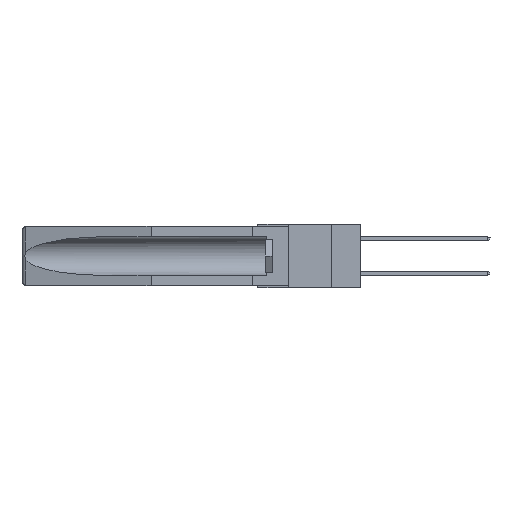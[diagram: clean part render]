
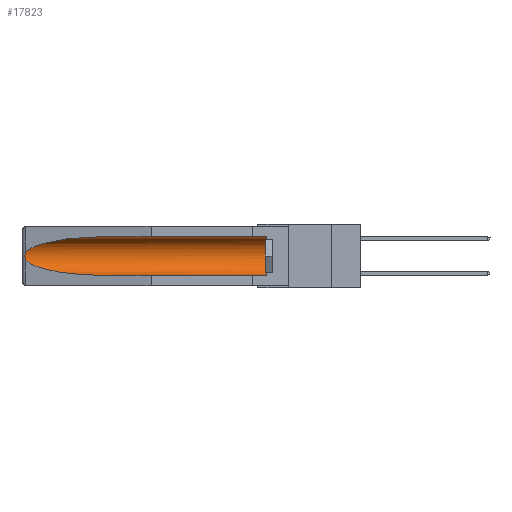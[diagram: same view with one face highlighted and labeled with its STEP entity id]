
A CAD part, left-side view. The second image highlights one B-rep face of the part: STEP entity #17823.
In plain terms, the highlighted cylindrical face has radius 2.857 mm (diameter 5.715 mm), a partial arc.
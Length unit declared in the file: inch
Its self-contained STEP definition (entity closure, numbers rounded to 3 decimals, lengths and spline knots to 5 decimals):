
#705 = DIRECTION ( 'NONE',  ( 0., -1., 0. ) ) ;
#1316 = CARTESIAN_POINT ( 'NONE',  ( 0.26537, 1.52718, -0.14972 ) ) ;
#1334 = VERTEX_POINT ( 'NONE', #18808 ) ;
#1489 = CARTESIAN_POINT ( 'NONE',  ( 0.2673, 1.5327, -0.16383 ) ) ;
#1999 = CARTESIAN_POINT ( 'NONE',  ( 0.155, 1.07973, -0.059 ) ) ;
#2081 = ORIENTED_EDGE ( 'NONE', *, *, #20982, .T. ) ;
#2221 = CARTESIAN_POINT ( 'NONE',  ( 0.155, -0.30754, -0.059 ) ) ;
#3164 = ORIENTED_EDGE ( 'NONE', *, *, #6836, .T. ) ;
#3399 = CARTESIAN_POINT ( 'NONE',  ( 0.2675, 1.53308, -0.16763 ) ) ;
#3469 = CARTESIAN_POINT ( 'NONE',  ( 0.2675, 1.53308, -0.17534 ) ) ;
#3472 = CARTESIAN_POINT ( 'NONE',  ( 0.155, 1.07973, -0.284 ) ) ;
#4184 = CARTESIAN_POINT ( 'NONE',  ( 0.155, -0.30754, -0.284 ) ) ;
#4378 = VERTEX_POINT ( 'NONE', #1999 ) ;
#4438 = CARTESIAN_POINT ( 'NONE',  ( 0.155, -0.30754, -0.1715 ) ) ;
#5436 = CARTESIAN_POINT ( 'NONE',  ( 0.2673, 1.53269, -0.17917 ) ) ;
#5707 =( BOUNDED_CURVE ( )  B_SPLINE_CURVE ( 3, ( #8137, #16280, #16543, #6509 ),
 .UNSPECIFIED., .F., .F. ) 
 B_SPLINE_CURVE_WITH_KNOTS ( ( 4, 4 ),
 ( 0.1948, 1.5708 ),
 .UNSPECIFIED. ) 
 CURVE ( )  GEOMETRIC_REPRESENTATION_ITEM ( )  RATIONAL_B_SPLINE_CURVE ( ( 1., 0.848, 0.848, 1. ) ) 
 REPRESENTATION_ITEM ( '' )  );
#6186 = EDGE_LOOP ( 'NONE', ( #16574, #25007, #3164, #14353, #10089, #2081 ) ) ;
#6472 = B_SPLINE_CURVE_WITH_KNOTS ( 'NONE', 3,
 ( #10465, #12458, #18932, #1489, #3399, #3469, #5436, #19088, #20959, #7041 ),
 .UNSPECIFIED., .F., .F.,
 ( 4, 2, 2, 2, 4 ),
 ( 0., 0.00029, 0.00058, 0.00087, 0.00117 ),
 .UNSPECIFIED. ) ;
#6509 = CARTESIAN_POINT ( 'NONE',  ( 0.155, 1.07973, -0.284 ) ) ;
#6632 = DIRECTION ( 'NONE',  ( 0., 1., 0. ) ) ;
#6836 = EDGE_CURVE ( 'NONE', #25185, #20317, #5707, .T. ) ;
#7041 = CARTESIAN_POINT ( 'NONE',  ( 0.26537, 1.52718, -0.19328 ) ) ;
#8137 = CARTESIAN_POINT ( 'NONE',  ( 0.26537, 1.52718, -0.19328 ) ) ;
#10089 = ORIENTED_EDGE ( 'NONE', *, *, #22306, .T. ) ;
#10140 = FACE_OUTER_BOUND ( 'NONE', #6186, .T. ) ;
#10465 = CARTESIAN_POINT ( 'NONE',  ( 0.26537, 1.52718, -0.14972 ) ) ;
#10828 = LINE ( 'NONE', #4184, #15139 ) ;
#12458 = CARTESIAN_POINT ( 'NONE',  ( 0.26597, 1.52961, -0.15275 ) ) ;
#13506 = EDGE_CURVE ( 'NONE', #17759, #25185, #6472, .T. ) ;
#14353 = ORIENTED_EDGE ( 'NONE', *, *, #17317, .F. ) ;
#14412 = DIRECTION ( 'NONE',  ( 0., 0., 1. ) ) ;
#14852 = CARTESIAN_POINT ( 'NONE',  ( 0.155, 1.07973, -0.059 ) ) ;
#15095 = CARTESIAN_POINT ( 'NONE',  ( 0.155, 0.126, -0.284 ) ) ;
#15120 = CIRCLE ( 'NONE', #21218, 0.1125 ) ;
#15139 = VECTOR ( 'NONE', #19806, 39.37008 ) ;
#15794 = AXIS2_PLACEMENT_3D ( 'NONE', #4438, #6632, #16234 ) ;
#16234 = DIRECTION ( 'NONE',  ( 0., 0., 1. ) ) ;
#16280 = CARTESIAN_POINT ( 'NONE',  ( 0.25451, 1.48313, -0.24835 ) ) ;
#16395 = CARTESIAN_POINT ( 'NONE',  ( 0.26537, 1.52718, -0.19328 ) ) ;
#16468 = CARTESIAN_POINT ( 'NONE',  ( 0.21114, 1.30732, -0.059 ) ) ;
#16543 = CARTESIAN_POINT ( 'NONE',  ( 0.21114, 1.30732, -0.284 ) ) ;
#16574 = ORIENTED_EDGE ( 'NONE', *, *, #17776, .T. ) ;
#17317 = EDGE_CURVE ( 'NONE', #19326, #20317, #10828, .T. ) ;
#17759 = VERTEX_POINT ( 'NONE', #24000 ) ;
#17776 = EDGE_CURVE ( 'NONE', #4378, #17759, #20892, .T. ) ;
#17820 = CYLINDRICAL_SURFACE ( 'NONE', #15794, 0.1125 ) ;
#17823 = ADVANCED_FACE ( 'NONE', ( #10140 ), #17820, .F. ) ;
#17859 = DIRECTION ( 'NONE',  ( 0., 1., 0. ) ) ;
#18218 = VECTOR ( 'NONE', #17859, 39.37008 ) ;
#18233 = CARTESIAN_POINT ( 'NONE',  ( 0.155, 0.126, -0.1715 ) ) ;
#18808 = CARTESIAN_POINT ( 'NONE',  ( 0.155, 0.126, -0.059 ) ) ;
#18837 = LINE ( 'NONE', #2221, #18218 ) ;
#18932 = CARTESIAN_POINT ( 'NONE',  ( 0.26654, 1.53092, -0.15636 ) ) ;
#19088 = CARTESIAN_POINT ( 'NONE',  ( 0.26655, 1.53094, -0.18657 ) ) ;
#19326 = VERTEX_POINT ( 'NONE', #15095 ) ;
#19806 = DIRECTION ( 'NONE',  ( 0., 1., 0. ) ) ;
#20317 = VERTEX_POINT ( 'NONE', #3472 ) ;
#20892 =( BOUNDED_CURVE ( )  B_SPLINE_CURVE ( 3, ( #14852, #16468, #22740, #1316 ),
 .UNSPECIFIED., .F., .F. ) 
 B_SPLINE_CURVE_WITH_KNOTS ( ( 4, 4 ),
 ( 4.71239, 6.08839 ),
 .UNSPECIFIED. ) 
 CURVE ( )  GEOMETRIC_REPRESENTATION_ITEM ( )  RATIONAL_B_SPLINE_CURVE ( ( 1., 0.848, 0.848, 1. ) ) 
 REPRESENTATION_ITEM ( '' )  );
#20959 = CARTESIAN_POINT ( 'NONE',  ( 0.26597, 1.5296, -0.19026 ) ) ;
#20982 = EDGE_CURVE ( 'NONE', #1334, #4378, #18837, .T. ) ;
#21218 = AXIS2_PLACEMENT_3D ( 'NONE', #18233, #705, #14412 ) ;
#22306 = EDGE_CURVE ( 'NONE', #19326, #1334, #15120, .T. ) ;
#22740 = CARTESIAN_POINT ( 'NONE',  ( 0.25451, 1.48313, -0.09465 ) ) ;
#24000 = CARTESIAN_POINT ( 'NONE',  ( 0.26537, 1.52718, -0.14972 ) ) ;
#25007 = ORIENTED_EDGE ( 'NONE', *, *, #13506, .T. ) ;
#25185 = VERTEX_POINT ( 'NONE', #16395 ) ;
